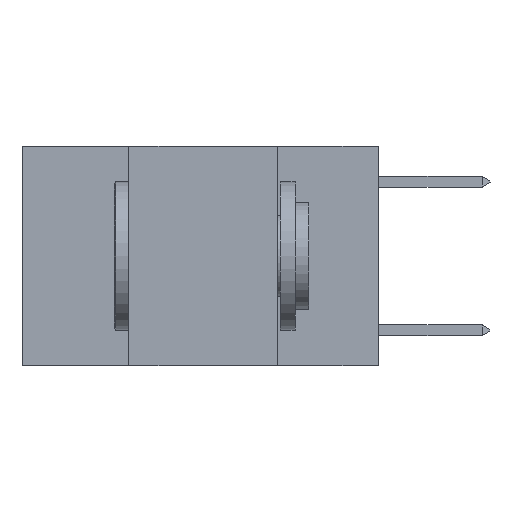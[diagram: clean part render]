
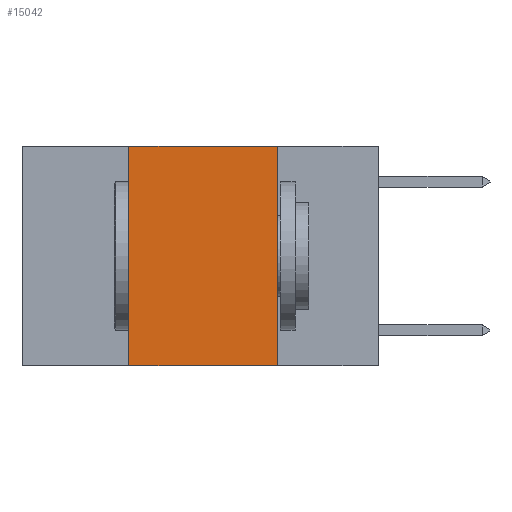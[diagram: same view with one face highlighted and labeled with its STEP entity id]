
A CAD part, left-side view. The second image highlights one B-rep face of the part: STEP entity #15042.
In plain terms, the highlighted planar face has unit normal (-1, 0, 0).
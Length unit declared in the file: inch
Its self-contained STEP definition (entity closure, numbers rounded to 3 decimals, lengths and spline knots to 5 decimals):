
#949 = ORIENTED_EDGE ( 'NONE', *, *, #14168, .F. ) ;
#1960 = VERTEX_POINT ( 'NONE', #15551 ) ;
#2377 = LINE ( 'NONE', #13013, #5770 ) ;
#3236 = ORIENTED_EDGE ( 'NONE', *, *, #15113, .F. ) ;
#3432 = CARTESIAN_POINT ( 'NONE',  ( 0., 0.42, 0. ) ) ;
#4560 = DIRECTION ( 'NONE',  ( 1., 0., 0. ) ) ;
#5643 = ORIENTED_EDGE ( 'NONE', *, *, #9008, .T. ) ;
#5770 = VECTOR ( 'NONE', #17777, 39.37008 ) ;
#6388 = VERTEX_POINT ( 'NONE', #7904 ) ;
#6608 = AXIS2_PLACEMENT_3D ( 'NONE', #19094, #4560, #15999 ) ;
#7162 = EDGE_CURVE ( 'NONE', #17242, #1960, #12878, .T. ) ;
#7904 = CARTESIAN_POINT ( 'NONE',  ( 0., 0.17, -0.37 ) ) ;
#9008 = EDGE_CURVE ( 'NONE', #17242, #6388, #9461, .T. ) ;
#9461 = LINE ( 'NONE', #11704, #13801 ) ;
#10332 = CARTESIAN_POINT ( 'NONE',  ( 0., 0.42, -0.37 ) ) ;
#11704 = CARTESIAN_POINT ( 'NONE',  ( 0., 0.6, -0.37 ) ) ;
#12012 = DIRECTION ( 'NONE',  ( 0., -1., 0. ) ) ;
#12878 = LINE ( 'NONE', #3432, #16105 ) ;
#13013 = CARTESIAN_POINT ( 'NONE',  ( 0., 0.6, 0. ) ) ;
#13536 = CARTESIAN_POINT ( 'NONE',  ( 0., 0.17, 0. ) ) ;
#13552 = VECTOR ( 'NONE', #20014, 39.37008 ) ;
#13605 = VERTEX_POINT ( 'NONE', #17217 ) ;
#13801 = VECTOR ( 'NONE', #12012, 39.37008 ) ;
#13968 = EDGE_LOOP ( 'NONE', ( #949, #3236, #19243, #5643 ) ) ;
#14168 = EDGE_CURVE ( 'NONE', #13605, #6388, #14559, .T. ) ;
#14409 = PLANE ( 'NONE',  #6608 ) ;
#14559 = LINE ( 'NONE', #13536, #13552 ) ;
#15042 = ADVANCED_FACE ( 'NONE', ( #16003 ), #14409, .F. ) ;
#15113 = EDGE_CURVE ( 'NONE', #1960, #13605, #2377, .T. ) ;
#15551 = CARTESIAN_POINT ( 'NONE',  ( 0., 0.42, 0. ) ) ;
#15999 = DIRECTION ( 'NONE',  ( 0., 0., -1. ) ) ;
#16003 = FACE_OUTER_BOUND ( 'NONE', #13968, .T. ) ;
#16105 = VECTOR ( 'NONE', #17846, 39.37008 ) ;
#17217 = CARTESIAN_POINT ( 'NONE',  ( 0., 0.17, 0. ) ) ;
#17242 = VERTEX_POINT ( 'NONE', #10332 ) ;
#17777 = DIRECTION ( 'NONE',  ( 0., -1., 0. ) ) ;
#17846 = DIRECTION ( 'NONE',  ( 0., 0., 1. ) ) ;
#19094 = CARTESIAN_POINT ( 'NONE',  ( 0., 0.6, 0. ) ) ;
#19243 = ORIENTED_EDGE ( 'NONE', *, *, #7162, .F. ) ;
#20014 = DIRECTION ( 'NONE',  ( 0., 0., -1. ) ) ;
